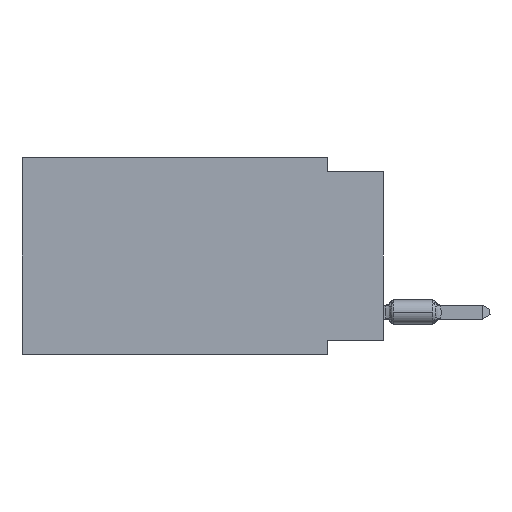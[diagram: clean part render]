
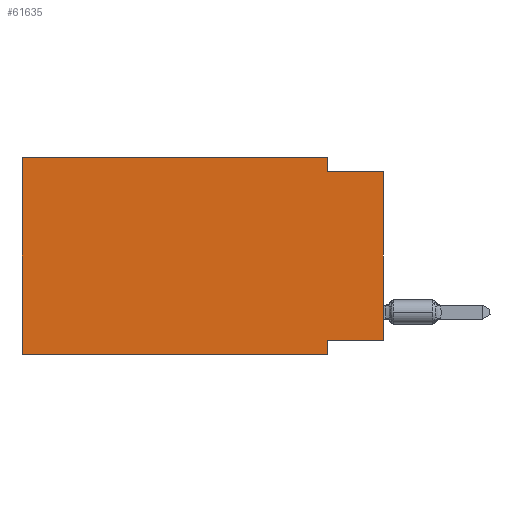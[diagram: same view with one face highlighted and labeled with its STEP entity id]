
A CAD part, left-side view. The second image highlights one B-rep face of the part: STEP entity #61635.
In plain terms, the highlighted planar face has unit normal (-1, 0, 0).
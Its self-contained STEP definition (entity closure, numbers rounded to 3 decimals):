
#831 = VERTEX_POINT ( 'NONE', #46813 ) ;
#4003 = EDGE_CURVE ( 'NONE', #38136, #44874, #45410, .T. ) ;
#4283 = CARTESIAN_POINT ( 'NONE',  ( 0., 2.54, -8.255 ) ) ;
#4499 = ORIENTED_EDGE ( 'NONE', *, *, #20817, .F. ) ;
#5399 = CARTESIAN_POINT ( 'NONE',  ( 0., 0., 0. ) ) ;
#6120 = CARTESIAN_POINT ( 'NONE',  ( 0., 16.383, -8.89 ) ) ;
#9804 = DIRECTION ( 'NONE',  ( 0., -1., 0. ) ) ;
#10746 = EDGE_CURVE ( 'NONE', #40476, #35900, #56568, .T. ) ;
#10862 = ORIENTED_EDGE ( 'NONE', *, *, #42514, .F. ) ;
#11955 = ORIENTED_EDGE ( 'NONE', *, *, #45008, .T. ) ;
#12433 = AXIS2_PLACEMENT_3D ( 'NONE', #32975, #58726, #53233 ) ;
#13295 = ORIENTED_EDGE ( 'NONE', *, *, #40064, .T. ) ;
#14760 = VECTOR ( 'NONE', #51235, 1000. ) ;
#14799 = VECTOR ( 'NONE', #61288, 1000. ) ;
#15002 = ORIENTED_EDGE ( 'NONE', *, *, #35249, .F. ) ;
#15189 = CARTESIAN_POINT ( 'NONE',  ( 0., 16.383, -8.89 ) ) ;
#15276 = DIRECTION ( 'NONE',  ( 0., 1., 0. ) ) ;
#15953 = LINE ( 'NONE', #67099, #48203 ) ;
#16131 = CARTESIAN_POINT ( 'NONE',  ( 0., 16.383, 0. ) ) ;
#20817 = EDGE_CURVE ( 'NONE', #22618, #38136, #41365, .T. ) ;
#21186 = VERTEX_POINT ( 'NONE', #15189 ) ;
#22618 = VERTEX_POINT ( 'NONE', #34873 ) ;
#23389 = CARTESIAN_POINT ( 'NONE',  ( 0., 2.54, 0. ) ) ;
#25001 = LINE ( 'NONE', #6120, #40824 ) ;
#27349 = VECTOR ( 'NONE', #67820, 1000. ) ;
#29146 = ORIENTED_EDGE ( 'NONE', *, *, #36241, .F. ) ;
#29960 = CARTESIAN_POINT ( 'NONE',  ( 0., 2.54, -8.89 ) ) ;
#30245 = EDGE_LOOP ( 'NONE', ( #11955, #10862, #34191, #29146, #15002, #13295, #66751, #4499 ) ) ;
#30391 = LINE ( 'NONE', #35855, #14799 ) ;
#30795 = CARTESIAN_POINT ( 'NONE',  ( 0., 2.54, 0. ) ) ;
#32256 = DIRECTION ( 'NONE',  ( 0., 0., 1. ) ) ;
#32975 = CARTESIAN_POINT ( 'NONE',  ( 0., 16.383, 0. ) ) ;
#34191 = ORIENTED_EDGE ( 'NONE', *, *, #10746, .F. ) ;
#34873 = CARTESIAN_POINT ( 'NONE',  ( 0., 0., -8.255 ) ) ;
#35249 = EDGE_CURVE ( 'NONE', #21186, #831, #63142, .T. ) ;
#35855 = CARTESIAN_POINT ( 'NONE',  ( 0., 0., -0.635 ) ) ;
#35900 = VERTEX_POINT ( 'NONE', #44859 ) ;
#36241 = EDGE_CURVE ( 'NONE', #831, #40476, #15953, .T. ) ;
#38136 = VERTEX_POINT ( 'NONE', #4283 ) ;
#40064 = EDGE_CURVE ( 'NONE', #21186, #44874, #25001, .T. ) ;
#40476 = VERTEX_POINT ( 'NONE', #23389 ) ;
#40824 = VECTOR ( 'NONE', #58290, 1000. ) ;
#41365 = LINE ( 'NONE', #62301, #62311 ) ;
#42072 = CARTESIAN_POINT ( 'NONE',  ( 0., 0., -0.635 ) ) ;
#42514 = EDGE_CURVE ( 'NONE', #35900, #62356, #30391, .T. ) ;
#44859 = CARTESIAN_POINT ( 'NONE',  ( 0., 2.54, -0.635 ) ) ;
#44874 = VERTEX_POINT ( 'NONE', #44911 ) ;
#44911 = CARTESIAN_POINT ( 'NONE',  ( 0., 2.54, -8.89 ) ) ;
#45008 = EDGE_CURVE ( 'NONE', #22618, #62356, #46586, .T. ) ;
#45410 = LINE ( 'NONE', #29960, #14760 ) ;
#46586 = LINE ( 'NONE', #5399, #62040 ) ;
#46813 = CARTESIAN_POINT ( 'NONE',  ( 0., 16.383, 0. ) ) ;
#48203 = VECTOR ( 'NONE', #9804, 1000. ) ;
#51235 = DIRECTION ( 'NONE',  ( 0., 0., -1. ) ) ;
#53233 = DIRECTION ( 'NONE',  ( 0., 0., -1. ) ) ;
#56568 = LINE ( 'NONE', #30795, #27349 ) ;
#58290 = DIRECTION ( 'NONE',  ( 0., -1., 0. ) ) ;
#58726 = DIRECTION ( 'NONE',  ( 1., 0., 0. ) ) ;
#61288 = DIRECTION ( 'NONE',  ( 0., -1., 0. ) ) ;
#61635 = ADVANCED_FACE ( 'NONE', ( #63852 ), #63158, .F. ) ;
#62040 = VECTOR ( 'NONE', #67497, 1000. ) ;
#62301 = CARTESIAN_POINT ( 'NONE',  ( 0., 0., -8.255 ) ) ;
#62311 = VECTOR ( 'NONE', #15276, 1000. ) ;
#62328 = VECTOR ( 'NONE', #32256, 1000. ) ;
#62356 = VERTEX_POINT ( 'NONE', #42072 ) ;
#63142 = LINE ( 'NONE', #16131, #62328 ) ;
#63158 = PLANE ( 'NONE',  #12433 ) ;
#63852 = FACE_OUTER_BOUND ( 'NONE', #30245, .T. ) ;
#66751 = ORIENTED_EDGE ( 'NONE', *, *, #4003, .F. ) ;
#67099 = CARTESIAN_POINT ( 'NONE',  ( 0., 16.383, 0. ) ) ;
#67497 = DIRECTION ( 'NONE',  ( 0., 0., 1. ) ) ;
#67820 = DIRECTION ( 'NONE',  ( 0., 0., -1. ) ) ;
